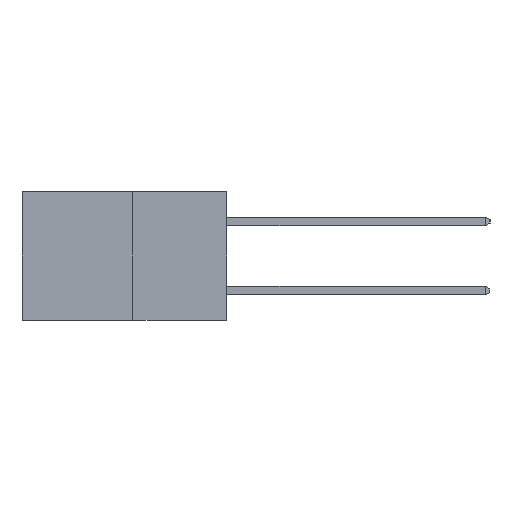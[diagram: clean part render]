
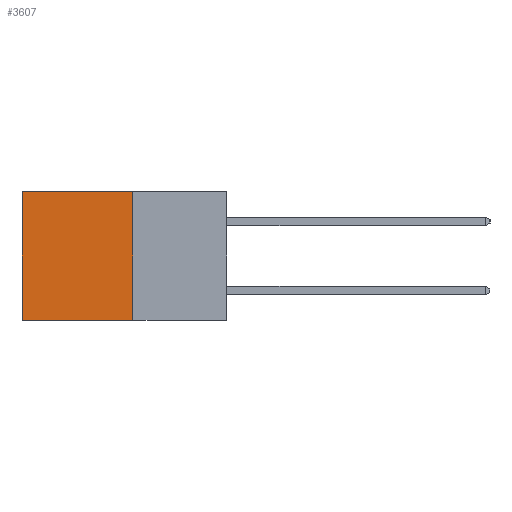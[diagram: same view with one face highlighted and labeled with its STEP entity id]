
A CAD part, left-side view. The second image highlights one B-rep face of the part: STEP entity #3607.
In plain terms, the highlighted planar face has unit normal (-1, 0, 0).
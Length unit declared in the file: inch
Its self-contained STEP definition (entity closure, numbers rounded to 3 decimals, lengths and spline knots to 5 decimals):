
#10 = CARTESIAN_POINT ( 'NONE',  ( 0.277, 0.59, 0. ) ) ;
#189 = CARTESIAN_POINT ( 'NONE',  ( 0.277, 0.27, -0.37 ) ) ;
#194 = VERTEX_POINT ( 'NONE', #8902 ) ;
#221 = CARTESIAN_POINT ( 'NONE',  ( 0.277, 0.59, -0.37 ) ) ;
#594 = FACE_OUTER_BOUND ( 'NONE', #1860, .T. ) ;
#1026 = DIRECTION ( 'NONE',  ( 1., 0., 0. ) ) ;
#1052 = CARTESIAN_POINT ( 'NONE',  ( 0.277, 0.27, -0.37 ) ) ;
#1096 = LINE ( 'NONE', #4678, #4845 ) ;
#1340 = VECTOR ( 'NONE', #2346, 39.37008 ) ;
#1860 = EDGE_LOOP ( 'NONE', ( #4939, #4946, #4954, #4987 ) ) ;
#2346 = DIRECTION ( 'NONE',  ( 0., 1., 0. ) ) ;
#2763 = EDGE_CURVE ( 'NONE', #7747, #8178, #6394, .T. ) ;
#3607 = ADVANCED_FACE ( 'NONE', ( #594 ), #5236, .F. ) ;
#3812 = DIRECTION ( 'NONE',  ( 0., 1., 0. ) ) ;
#3856 = CARTESIAN_POINT ( 'NONE',  ( 0.277, 0.27, 0. ) ) ;
#4678 = CARTESIAN_POINT ( 'NONE',  ( 0.277, 0.27, -0.37 ) ) ;
#4845 = VECTOR ( 'NONE', #7528, 39.37008 ) ;
#4899 = VERTEX_POINT ( 'NONE', #4901 ) ;
#4901 = CARTESIAN_POINT ( 'NONE',  ( 0.277, 0.27, 0. ) ) ;
#4939 = ORIENTED_EDGE ( 'NONE', *, *, #2763, .T. ) ;
#4946 = ORIENTED_EDGE ( 'NONE', *, *, #8158, .F. ) ;
#4954 = ORIENTED_EDGE ( 'NONE', *, *, #8179, .F. ) ;
#4957 = EDGE_CURVE ( 'NONE', #4899, #7747, #5245, .T. ) ;
#4987 = ORIENTED_EDGE ( 'NONE', *, *, #4957, .T. ) ;
#4993 = VECTOR ( 'NONE', #3812, 39.37008 ) ;
#5236 = PLANE ( 'NONE',  #7619 ) ;
#5245 = LINE ( 'NONE', #3856, #4993 ) ;
#5322 = LINE ( 'NONE', #189, #1340 ) ;
#6394 = LINE ( 'NONE', #6580, #7767 ) ;
#6580 = CARTESIAN_POINT ( 'NONE',  ( 0.277, 0.59, -0.37 ) ) ;
#6854 = DIRECTION ( 'NONE',  ( 0., 0., -1. ) ) ;
#6955 = DIRECTION ( 'NONE',  ( 0., 0., -1. ) ) ;
#7528 = DIRECTION ( 'NONE',  ( 0., 0., -1. ) ) ;
#7619 = AXIS2_PLACEMENT_3D ( 'NONE', #1052, #1026, #6955 ) ;
#7747 = VERTEX_POINT ( 'NONE', #10 ) ;
#7767 = VECTOR ( 'NONE', #6854, 39.37008 ) ;
#8158 = EDGE_CURVE ( 'NONE', #194, #8178, #5322, .T. ) ;
#8178 = VERTEX_POINT ( 'NONE', #221 ) ;
#8179 = EDGE_CURVE ( 'NONE', #4899, #194, #1096, .T. ) ;
#8902 = CARTESIAN_POINT ( 'NONE',  ( 0.277, 0.27, -0.37 ) ) ;
